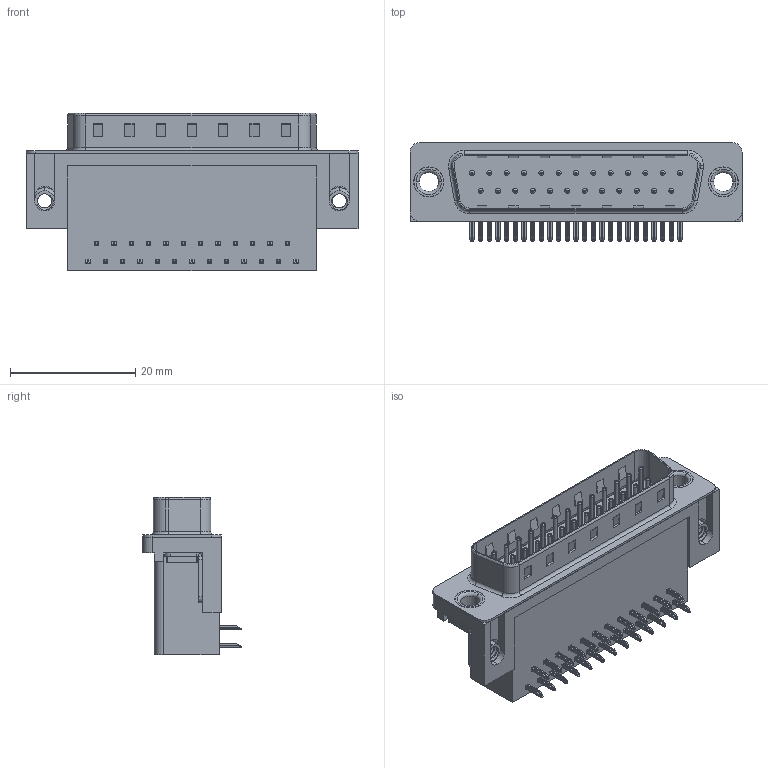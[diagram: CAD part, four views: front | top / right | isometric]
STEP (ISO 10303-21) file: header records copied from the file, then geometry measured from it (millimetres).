
FILE_DESCRIPTION (( 'STEP AP203' ), '1' );
FILE_NAME ('625-025-362-051.STEP', '2018-11-06T02:28:50', ( '' ), ( '' ), 'SwSTEP 2.0', 'SolidWorks 2016', '' );
FILE_SCHEMA (( 'CONFIG_CONTROL_DESIGN' ));
Length unit declared in the file: millimetre
Products named in the file (7): 625 Contact Bottom; 625 4-40 Threaded Board Mount; 625 Thru Hole Rivet; 625-025-362-051; 625 Housing_25 Socket; 625 Shell_25 Socket; 625 Contact Top
Assembly tree (31 placements, depth 2):
  625-025-362-051
    625 Housing_25 Socket
    625 Shell_25 Socket
    625 Contact Bottom  x12
    625 Contact Top  x13
    625 4-40 Threaded Board Mount  x2
    625 Thru Hole Rivet  x2
Bounding box: 53.04 x 15.73 x 25.16 mm (x, y, z)
Volume: 9163.1 mm3; surface area: 8917.6 mm2
Topology: 31 solids, 31 shells, 2257 faces, 5587 edges, 3451 vertices
Faces by surface type: plane 1407, cylinder 655, torus 189, bspline 6
Entity records: 22275 total; most frequent: CARTESIAN_POINT 4832, DIRECTION 3401, ORIENTED_EDGE 3252, EDGE_CURVE 1626, VECTOR 1147, LINE 1147, AXIS2_PLACEMENT_3D 1127, VERTEX_POINT 1043
